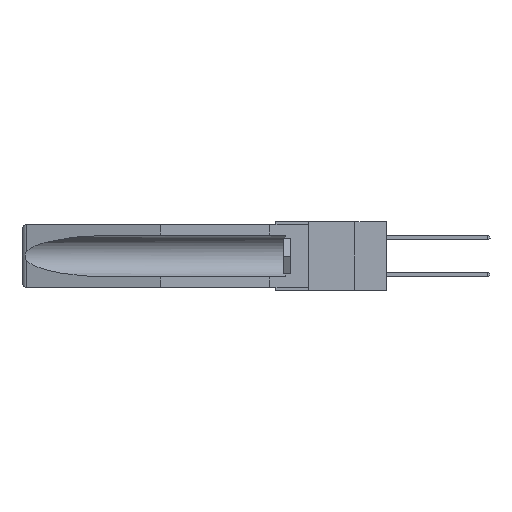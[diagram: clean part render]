
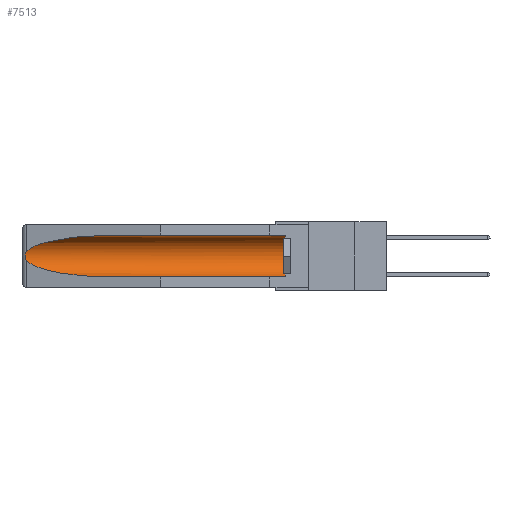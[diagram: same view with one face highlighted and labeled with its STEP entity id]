
A CAD part, left-side view. The second image highlights one B-rep face of the part: STEP entity #7513.
In plain terms, the highlighted cylindrical face has radius 2.857 mm (diameter 5.715 mm), a partial arc.
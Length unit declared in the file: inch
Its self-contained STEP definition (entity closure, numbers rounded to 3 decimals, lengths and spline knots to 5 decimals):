
#523 = B_SPLINE_CURVE_WITH_KNOTS ( 'NONE', 3,
 ( #26855, #6538, #19485, #4356, #23987, #6439, #16513, #1743, #12065, #12827 ),
 .UNSPECIFIED., .F., .F.,
 ( 4, 2, 2, 2, 4 ),
 ( 0., 0.00029, 0.00058, 0.00087, 0.00117 ),
 .UNSPECIFIED. ) ;
#1564 = LINE ( 'NONE', #1661, #28369 ) ;
#1661 = CARTESIAN_POINT ( 'NONE',  ( 0.155, -0.30754, -0.059 ) ) ;
#1743 = CARTESIAN_POINT ( 'NONE',  ( 0.26655, 1.53094, -0.18657 ) ) ;
#1927 = CARTESIAN_POINT ( 'NONE',  ( 0.155, 0.126, -0.059 ) ) ;
#3389 = CARTESIAN_POINT ( 'NONE',  ( 0.26537, 1.52718, -0.14972 ) ) ;
#3666 = VERTEX_POINT ( 'NONE', #22192 ) ;
#4356 = CARTESIAN_POINT ( 'NONE',  ( 0.2673, 1.5327, -0.16383 ) ) ;
#4917 =( BOUNDED_CURVE ( )  B_SPLINE_CURVE ( 3, ( #16158, #26398, #30943, #3389 ),
 .UNSPECIFIED., .F., .F. ) 
 B_SPLINE_CURVE_WITH_KNOTS ( ( 4, 4 ),
 ( 4.71239, 6.08839 ),
 .UNSPECIFIED. ) 
 CURVE ( )  GEOMETRIC_REPRESENTATION_ITEM ( )  RATIONAL_B_SPLINE_CURVE ( ( 1., 0.848, 0.848, 1. ) ) 
 REPRESENTATION_ITEM ( '' )  );
#5016 = CARTESIAN_POINT ( 'NONE',  ( 0.25451, 1.48313, -0.24835 ) ) ;
#5134 = VERTEX_POINT ( 'NONE', #23799 ) ;
#6439 = CARTESIAN_POINT ( 'NONE',  ( 0.2675, 1.53308, -0.17534 ) ) ;
#6538 = CARTESIAN_POINT ( 'NONE',  ( 0.26597, 1.52961, -0.15275 ) ) ;
#7017 = ORIENTED_EDGE ( 'NONE', *, *, #9040, .T. ) ;
#7305 = AXIS2_PLACEMENT_3D ( 'NONE', #9998, #12317, #22475 ) ;
#7503 = DIRECTION ( 'NONE',  ( 0., 0., 1. ) ) ;
#7513 = ADVANCED_FACE ( 'NONE', ( #32156 ), #9255, .F. ) ;
#7729 = DIRECTION ( 'NONE',  ( 0., -1., 0. ) ) ;
#7792 = CARTESIAN_POINT ( 'NONE',  ( 0.155, 0.126, -0.284 ) ) ;
#8006 = EDGE_CURVE ( 'NONE', #9493, #26190, #30544, .T. ) ;
#9040 = EDGE_CURVE ( 'NONE', #5134, #29081, #523, .T. ) ;
#9226 = DIRECTION ( 'NONE',  ( 0., 1., 0. ) ) ;
#9255 = CYLINDRICAL_SURFACE ( 'NONE', #7305, 0.1125 ) ;
#9493 = VERTEX_POINT ( 'NONE', #7792 ) ;
#9762 = CARTESIAN_POINT ( 'NONE',  ( 0.155, 1.07973, -0.284 ) ) ;
#9998 = CARTESIAN_POINT ( 'NONE',  ( 0.155, -0.30754, -0.1715 ) ) ;
#11361 = EDGE_CURVE ( 'NONE', #26190, #17709, #1564, .T. ) ;
#11454 = CARTESIAN_POINT ( 'NONE',  ( 0.26537, 1.52718, -0.19328 ) ) ;
#11579 = AXIS2_PLACEMENT_3D ( 'NONE', #17806, #7729, #7503 ) ;
#12065 = CARTESIAN_POINT ( 'NONE',  ( 0.26597, 1.5296, -0.19026 ) ) ;
#12105 = ORIENTED_EDGE ( 'NONE', *, *, #13888, .T. ) ;
#12211 = EDGE_CURVE ( 'NONE', #17709, #5134, #4917, .T. ) ;
#12317 = DIRECTION ( 'NONE',  ( 0., 1., 0. ) ) ;
#12827 = CARTESIAN_POINT ( 'NONE',  ( 0.26537, 1.52718, -0.19328 ) ) ;
#13888 = EDGE_CURVE ( 'NONE', #29081, #3666, #29779, .T. ) ;
#16158 = CARTESIAN_POINT ( 'NONE',  ( 0.155, 1.07973, -0.059 ) ) ;
#16402 = ORIENTED_EDGE ( 'NONE', *, *, #11361, .T. ) ;
#16513 = CARTESIAN_POINT ( 'NONE',  ( 0.2673, 1.53269, -0.17917 ) ) ;
#16547 = ORIENTED_EDGE ( 'NONE', *, *, #8006, .T. ) ;
#16972 = CARTESIAN_POINT ( 'NONE',  ( 0.155, 1.07973, -0.059 ) ) ;
#17709 = VERTEX_POINT ( 'NONE', #16972 ) ;
#17806 = CARTESIAN_POINT ( 'NONE',  ( 0.155, 0.126, -0.1715 ) ) ;
#18333 = ORIENTED_EDGE ( 'NONE', *, *, #12211, .T. ) ;
#19485 = CARTESIAN_POINT ( 'NONE',  ( 0.26654, 1.53092, -0.15636 ) ) ;
#20153 = EDGE_LOOP ( 'NONE', ( #18333, #7017, #12105, #30922, #16547, #16402 ) ) ;
#22070 = EDGE_CURVE ( 'NONE', #9493, #3666, #23748, .T. ) ;
#22192 = CARTESIAN_POINT ( 'NONE',  ( 0.155, 1.07973, -0.284 ) ) ;
#22224 = CARTESIAN_POINT ( 'NONE',  ( 0.26537, 1.52718, -0.19328 ) ) ;
#22475 = DIRECTION ( 'NONE',  ( 0., 0., 1. ) ) ;
#23748 = LINE ( 'NONE', #32519, #26119 ) ;
#23799 = CARTESIAN_POINT ( 'NONE',  ( 0.26537, 1.52718, -0.14972 ) ) ;
#23987 = CARTESIAN_POINT ( 'NONE',  ( 0.2675, 1.53308, -0.16763 ) ) ;
#24863 = CARTESIAN_POINT ( 'NONE',  ( 0.21114, 1.30732, -0.284 ) ) ;
#26119 = VECTOR ( 'NONE', #29643, 39.37008 ) ;
#26190 = VERTEX_POINT ( 'NONE', #1927 ) ;
#26398 = CARTESIAN_POINT ( 'NONE',  ( 0.21114, 1.30732, -0.059 ) ) ;
#26855 = CARTESIAN_POINT ( 'NONE',  ( 0.26537, 1.52718, -0.14972 ) ) ;
#28369 = VECTOR ( 'NONE', #9226, 39.37008 ) ;
#29081 = VERTEX_POINT ( 'NONE', #11454 ) ;
#29643 = DIRECTION ( 'NONE',  ( 0., 1., 0. ) ) ;
#29779 =( BOUNDED_CURVE ( )  B_SPLINE_CURVE ( 3, ( #22224, #5016, #24863, #9762 ),
 .UNSPECIFIED., .F., .F. ) 
 B_SPLINE_CURVE_WITH_KNOTS ( ( 4, 4 ),
 ( 0.1948, 1.5708 ),
 .UNSPECIFIED. ) 
 CURVE ( )  GEOMETRIC_REPRESENTATION_ITEM ( )  RATIONAL_B_SPLINE_CURVE ( ( 1., 0.848, 0.848, 1. ) ) 
 REPRESENTATION_ITEM ( '' )  );
#30544 = CIRCLE ( 'NONE', #11579, 0.1125 ) ;
#30922 = ORIENTED_EDGE ( 'NONE', *, *, #22070, .F. ) ;
#30943 = CARTESIAN_POINT ( 'NONE',  ( 0.25451, 1.48313, -0.09465 ) ) ;
#32156 = FACE_OUTER_BOUND ( 'NONE', #20153, .T. ) ;
#32519 = CARTESIAN_POINT ( 'NONE',  ( 0.155, -0.30754, -0.284 ) ) ;
